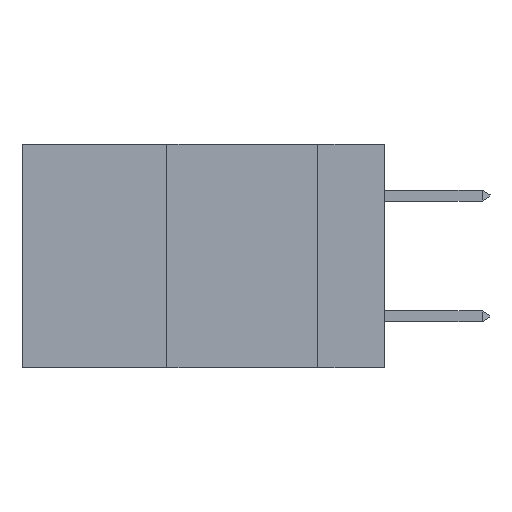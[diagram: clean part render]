
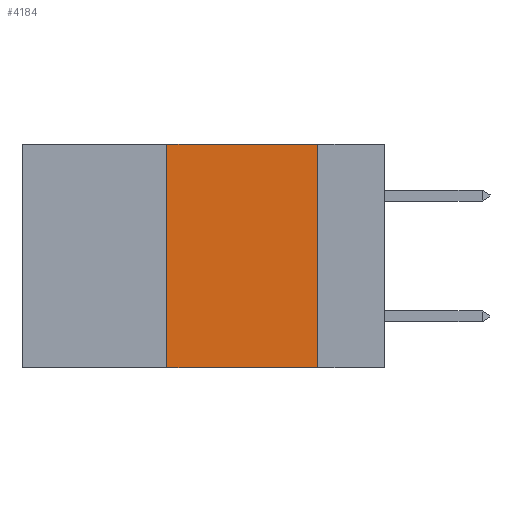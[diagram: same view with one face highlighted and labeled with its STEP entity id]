
A CAD part, left-side view. The second image highlights one B-rep face of the part: STEP entity #4184.
In plain terms, the highlighted planar face has unit normal (-1, 0, 0).
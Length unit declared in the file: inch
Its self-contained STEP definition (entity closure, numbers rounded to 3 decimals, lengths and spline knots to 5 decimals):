
#285 = VERTEX_POINT ( 'NONE', #12235 ) ;
#776 = DIRECTION ( 'NONE',  ( 0., -1., 0. ) ) ;
#1322 = CARTESIAN_POINT ( 'NONE',  ( 0., 0.6, 0. ) ) ;
#1323 = PLANE ( 'NONE',  #11629 ) ;
#1481 = VECTOR ( 'NONE', #9603, 39.37008 ) ;
#1631 = CARTESIAN_POINT ( 'NONE',  ( 0., 0.11, 0. ) ) ;
#3891 = EDGE_CURVE ( 'NONE', #12799, #9650, #6502, .T. ) ;
#3908 = LINE ( 'NONE', #7883, #11640 ) ;
#3950 = LINE ( 'NONE', #11158, #9187 ) ;
#4184 = ADVANCED_FACE ( 'NONE', ( #9357 ), #1323, .F. ) ;
#4542 = DIRECTION ( 'NONE',  ( 1., 0., 0. ) ) ;
#4596 = CARTESIAN_POINT ( 'NONE',  ( 0., 0.11, 0. ) ) ;
#4783 = CARTESIAN_POINT ( 'NONE',  ( 0., 0.6, 0. ) ) ;
#4923 = EDGE_CURVE ( 'NONE', #7508, #285, #3950, .T. ) ;
#5640 = DIRECTION ( 'NONE',  ( 0., 0., -1. ) ) ;
#5945 = CARTESIAN_POINT ( 'NONE',  ( 0., 0.36, 0. ) ) ;
#6289 = EDGE_CURVE ( 'NONE', #7508, #12799, #3908, .T. ) ;
#6356 = VECTOR ( 'NONE', #776, 39.37008 ) ;
#6502 = LINE ( 'NONE', #4783, #6356 ) ;
#7214 = ORIENTED_EDGE ( 'NONE', *, *, #3891, .F. ) ;
#7262 = CARTESIAN_POINT ( 'NONE',  ( 0., 0.36, -0.37 ) ) ;
#7508 = VERTEX_POINT ( 'NONE', #7262 ) ;
#7840 = DIRECTION ( 'NONE',  ( 0., 0., 1. ) ) ;
#7883 = CARTESIAN_POINT ( 'NONE',  ( 0., 0.36, 0. ) ) ;
#7920 = ORIENTED_EDGE ( 'NONE', *, *, #8745, .F. ) ;
#8745 = EDGE_CURVE ( 'NONE', #9650, #285, #11422, .T. ) ;
#9066 = DIRECTION ( 'NONE',  ( 0., -1., 0. ) ) ;
#9187 = VECTOR ( 'NONE', #9066, 39.37008 ) ;
#9357 = FACE_OUTER_BOUND ( 'NONE', #12188, .T. ) ;
#9603 = DIRECTION ( 'NONE',  ( 0., 0., -1. ) ) ;
#9650 = VERTEX_POINT ( 'NONE', #1631 ) ;
#10650 = ORIENTED_EDGE ( 'NONE', *, *, #6289, .F. ) ;
#11158 = CARTESIAN_POINT ( 'NONE',  ( 0., 0.6, -0.37 ) ) ;
#11422 = LINE ( 'NONE', #4596, #1481 ) ;
#11629 = AXIS2_PLACEMENT_3D ( 'NONE', #1322, #4542, #5640 ) ;
#11640 = VECTOR ( 'NONE', #7840, 39.37008 ) ;
#12188 = EDGE_LOOP ( 'NONE', ( #7920, #7214, #10650, #12202 ) ) ;
#12202 = ORIENTED_EDGE ( 'NONE', *, *, #4923, .T. ) ;
#12235 = CARTESIAN_POINT ( 'NONE',  ( 0., 0.11, -0.37 ) ) ;
#12799 = VERTEX_POINT ( 'NONE', #5945 ) ;
